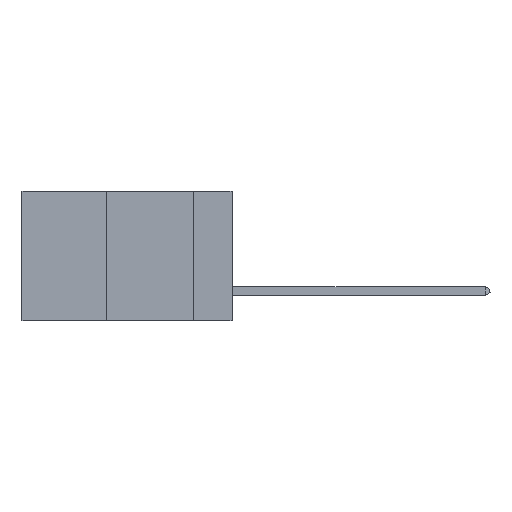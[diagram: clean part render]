
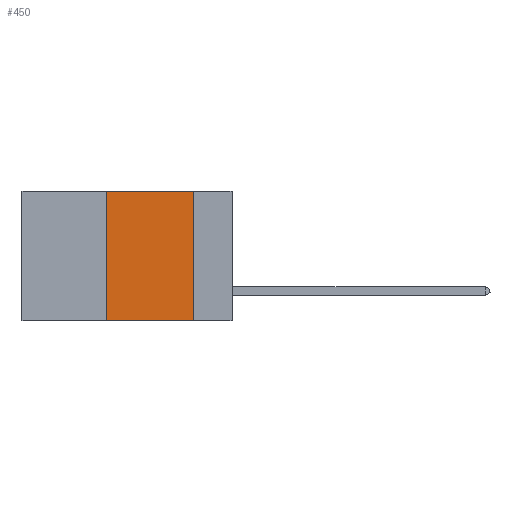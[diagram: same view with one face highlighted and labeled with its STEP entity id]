
A CAD part, left-side view. The second image highlights one B-rep face of the part: STEP entity #450.
In plain terms, the highlighted planar face has unit normal (-1, 0, 0).
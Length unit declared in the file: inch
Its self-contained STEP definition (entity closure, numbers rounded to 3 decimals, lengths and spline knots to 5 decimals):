
#162 = CARTESIAN_POINT ( 'NONE',  ( 0., 0.6, 0. ) ) ;
#240 = ORIENTED_EDGE ( 'NONE', *, *, #9809, .F. ) ;
#319 = VERTEX_POINT ( 'NONE', #1766 ) ;
#450 = ADVANCED_FACE ( 'NONE', ( #5867 ), #8712, .F. ) ;
#1191 = DIRECTION ( 'NONE',  ( 0., 0., -1. ) ) ;
#1330 = LINE ( 'NONE', #7819, #12085 ) ;
#1369 = CARTESIAN_POINT ( 'NONE',  ( 0., 0.6, 0. ) ) ;
#1449 = VECTOR ( 'NONE', #1191, 39.37008 ) ;
#1450 = LINE ( 'NONE', #1369, #6252 ) ;
#1725 = ORIENTED_EDGE ( 'NONE', *, *, #11315, .T. ) ;
#1766 = CARTESIAN_POINT ( 'NONE',  ( 0., 0.36, 0. ) ) ;
#3064 = DIRECTION ( 'NONE',  ( 0., 0., 1. ) ) ;
#4010 = CARTESIAN_POINT ( 'NONE',  ( 0., 0.11, 0. ) ) ;
#4163 = LINE ( 'NONE', #4010, #1449 ) ;
#5398 = VERTEX_POINT ( 'NONE', #9153 ) ;
#5831 = EDGE_CURVE ( 'NONE', #10529, #5398, #4163, .T. ) ;
#5867 = FACE_OUTER_BOUND ( 'NONE', #9519, .T. ) ;
#6252 = VECTOR ( 'NONE', #9105, 39.37008 ) ;
#7585 = ORIENTED_EDGE ( 'NONE', *, *, #5831, .F. ) ;
#7654 = CARTESIAN_POINT ( 'NONE',  ( 0., 0.11, 0. ) ) ;
#7819 = CARTESIAN_POINT ( 'NONE',  ( 0., 0.36, 0. ) ) ;
#8631 = EDGE_CURVE ( 'NONE', #10965, #319, #1330, .T. ) ;
#8712 = PLANE ( 'NONE',  #10219 ) ;
#8935 = CARTESIAN_POINT ( 'NONE',  ( 0., 0.6, -0.37 ) ) ;
#9032 = LINE ( 'NONE', #8935, #12015 ) ;
#9105 = DIRECTION ( 'NONE',  ( 0., -1., 0. ) ) ;
#9153 = CARTESIAN_POINT ( 'NONE',  ( 0., 0.11, -0.37 ) ) ;
#9226 = CARTESIAN_POINT ( 'NONE',  ( 0., 0.36, -0.37 ) ) ;
#9519 = EDGE_LOOP ( 'NONE', ( #7585, #240, #11854, #1725 ) ) ;
#9809 = EDGE_CURVE ( 'NONE', #319, #10529, #1450, .T. ) ;
#9816 = DIRECTION ( 'NONE',  ( 1., 0., 0. ) ) ;
#10219 = AXIS2_PLACEMENT_3D ( 'NONE', #162, #9816, #10586 ) ;
#10529 = VERTEX_POINT ( 'NONE', #7654 ) ;
#10586 = DIRECTION ( 'NONE',  ( 0., 0., -1. ) ) ;
#10823 = DIRECTION ( 'NONE',  ( 0., -1., 0. ) ) ;
#10965 = VERTEX_POINT ( 'NONE', #9226 ) ;
#11315 = EDGE_CURVE ( 'NONE', #10965, #5398, #9032, .T. ) ;
#11854 = ORIENTED_EDGE ( 'NONE', *, *, #8631, .F. ) ;
#12015 = VECTOR ( 'NONE', #10823, 39.37008 ) ;
#12085 = VECTOR ( 'NONE', #3064, 39.37008 ) ;
